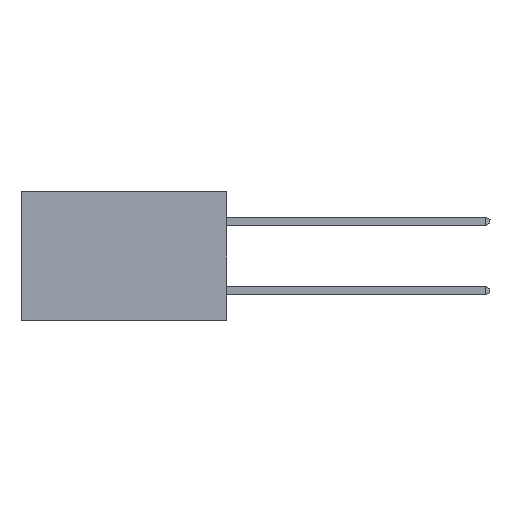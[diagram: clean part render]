
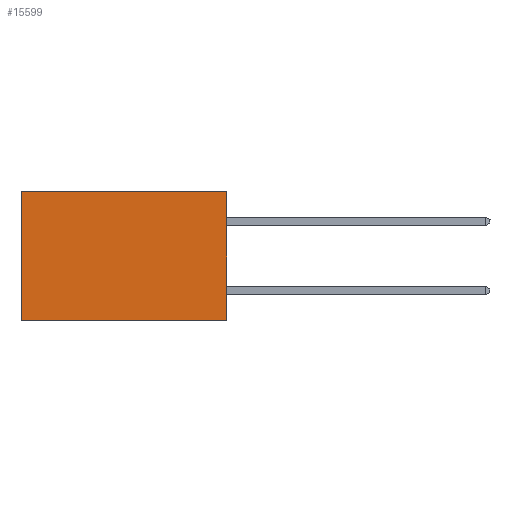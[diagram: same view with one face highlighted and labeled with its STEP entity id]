
A CAD part, left-side view. The second image highlights one B-rep face of the part: STEP entity #15599.
In plain terms, the highlighted planar face has unit normal (-1, 0, 0).
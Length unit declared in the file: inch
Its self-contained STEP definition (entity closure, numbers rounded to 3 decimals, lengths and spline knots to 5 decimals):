
#365 = AXIS2_PLACEMENT_3D ( 'NONE', #3481, #19644, #5845 ) ;
#2191 = DIRECTION ( 'NONE',  ( 0., 1., 0. ) ) ;
#3191 = VECTOR ( 'NONE', #2191, 39.37008 ) ;
#3481 = CARTESIAN_POINT ( 'NONE',  ( 0.277, 0., -0.37 ) ) ;
#3585 = EDGE_CURVE ( 'NONE', #8182, #16016, #4759, .T. ) ;
#4759 = LINE ( 'NONE', #21257, #10194 ) ;
#4913 = CARTESIAN_POINT ( 'NONE',  ( 0.277, 0.59, -0.37 ) ) ;
#5117 = VERTEX_POINT ( 'NONE', #11548 ) ;
#5552 = VERTEX_POINT ( 'NONE', #29016 ) ;
#5845 = DIRECTION ( 'NONE',  ( 0., 0., -1. ) ) ;
#7834 = EDGE_CURVE ( 'NONE', #5117, #16016, #27927, .T. ) ;
#7910 = VECTOR ( 'NONE', #26776, 39.37008 ) ;
#8182 = VERTEX_POINT ( 'NONE', #11409 ) ;
#8629 = LINE ( 'NONE', #17572, #7910 ) ;
#10194 = VECTOR ( 'NONE', #19440, 39.37008 ) ;
#10338 = ORIENTED_EDGE ( 'NONE', *, *, #3585, .F. ) ;
#11409 = CARTESIAN_POINT ( 'NONE',  ( 0.277, 0., -0.37 ) ) ;
#11548 = CARTESIAN_POINT ( 'NONE',  ( 0.277, 0.59, 0. ) ) ;
#12864 = EDGE_LOOP ( 'NONE', ( #24226, #10338, #19956, #26877 ) ) ;
#13736 = CARTESIAN_POINT ( 'NONE',  ( 0.277, 0., 0. ) ) ;
#14338 = VECTOR ( 'NONE', #26196, 39.37008 ) ;
#15599 = ADVANCED_FACE ( 'NONE', ( #28580 ), #17349, .F. ) ;
#16016 = VERTEX_POINT ( 'NONE', #4913 ) ;
#17349 = PLANE ( 'NONE',  #365 ) ;
#17572 = CARTESIAN_POINT ( 'NONE',  ( 0.277, 0., -0.37 ) ) ;
#19440 = DIRECTION ( 'NONE',  ( 0., 1., 0. ) ) ;
#19545 = EDGE_CURVE ( 'NONE', #5552, #5117, #21618, .T. ) ;
#19644 = DIRECTION ( 'NONE',  ( 1., 0., 0. ) ) ;
#19956 = ORIENTED_EDGE ( 'NONE', *, *, #20717, .F. ) ;
#20717 = EDGE_CURVE ( 'NONE', #5552, #8182, #8629, .T. ) ;
#21257 = CARTESIAN_POINT ( 'NONE',  ( 0.277, 0., -0.37 ) ) ;
#21618 = LINE ( 'NONE', #13736, #3191 ) ;
#23894 = CARTESIAN_POINT ( 'NONE',  ( 0.277, 0.59, -0.37 ) ) ;
#24226 = ORIENTED_EDGE ( 'NONE', *, *, #7834, .T. ) ;
#26196 = DIRECTION ( 'NONE',  ( 0., 0., -1. ) ) ;
#26776 = DIRECTION ( 'NONE',  ( 0., 0., -1. ) ) ;
#26877 = ORIENTED_EDGE ( 'NONE', *, *, #19545, .T. ) ;
#27927 = LINE ( 'NONE', #23894, #14338 ) ;
#28580 = FACE_OUTER_BOUND ( 'NONE', #12864, .T. ) ;
#29016 = CARTESIAN_POINT ( 'NONE',  ( 0.277, 0., 0. ) ) ;
